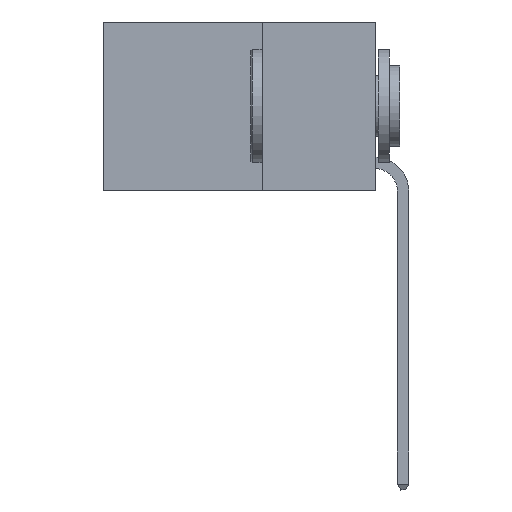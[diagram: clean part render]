
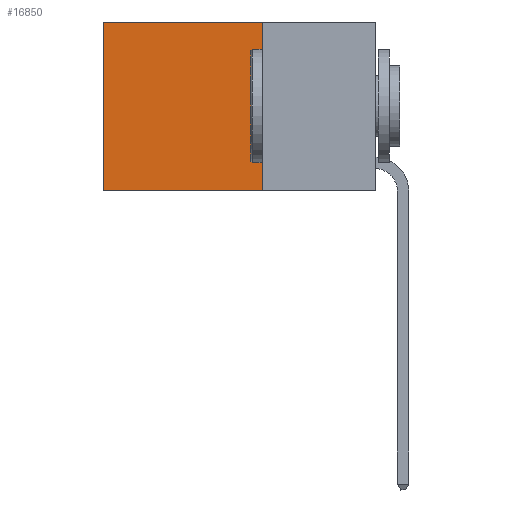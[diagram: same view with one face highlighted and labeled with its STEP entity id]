
A CAD part, left-side view. The second image highlights one B-rep face of the part: STEP entity #16850.
In plain terms, the highlighted planar face has unit normal (-1, 0, 0).
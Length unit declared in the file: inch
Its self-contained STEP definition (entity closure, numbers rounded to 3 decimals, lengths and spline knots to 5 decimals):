
#1317 = EDGE_CURVE ( 'NONE', #27462, #2827, #13480, .T. ) ;
#1613 = EDGE_CURVE ( 'NONE', #23934, #27462, #19766, .T. ) ;
#2827 = VERTEX_POINT ( 'NONE', #24064 ) ;
#3858 = CARTESIAN_POINT ( 'NONE',  ( 0.2625, 0.25, 0. ) ) ;
#4272 = LINE ( 'NONE', #3858, #9560 ) ;
#5053 = VECTOR ( 'NONE', #24504, 39.37008 ) ;
#6585 = DIRECTION ( 'NONE',  ( 0., 0., -1. ) ) ;
#6902 = ORIENTED_EDGE ( 'NONE', *, *, #8691, .T. ) ;
#7244 = CARTESIAN_POINT ( 'NONE',  ( 0.2625, 0.6, 0. ) ) ;
#8462 = DIRECTION ( 'NONE',  ( 0., 0., -1. ) ) ;
#8691 = EDGE_CURVE ( 'NONE', #23934, #18591, #4272, .T. ) ;
#9006 = PLANE ( 'NONE',  #9726 ) ;
#9560 = VECTOR ( 'NONE', #14703, 39.37008 ) ;
#9579 = VECTOR ( 'NONE', #8462, 39.37008 ) ;
#9649 = CARTESIAN_POINT ( 'NONE',  ( 0.2625, 0.6, 0. ) ) ;
#9726 = AXIS2_PLACEMENT_3D ( 'NONE', #11151, #21744, #6585 ) ;
#11151 = CARTESIAN_POINT ( 'NONE',  ( 0.2625, 0.25, 0. ) ) ;
#13480 = LINE ( 'NONE', #16049, #5053 ) ;
#13597 = CARTESIAN_POINT ( 'NONE',  ( 0.2625, 0.25, 0. ) ) ;
#14356 = DIRECTION ( 'NONE',  ( 0., 0., -1. ) ) ;
#14703 = DIRECTION ( 'NONE',  ( 0., 1., 0. ) ) ;
#14743 = ORIENTED_EDGE ( 'NONE', *, *, #21431, .T. ) ;
#15026 = CARTESIAN_POINT ( 'NONE',  ( 0.2625, 0.25, 0. ) ) ;
#16049 = CARTESIAN_POINT ( 'NONE',  ( 0.2625, 0.25, -0.37 ) ) ;
#16228 = LINE ( 'NONE', #9649, #24456 ) ;
#16850 = ADVANCED_FACE ( 'NONE', ( #24316 ), #9006, .F. ) ;
#16988 = EDGE_LOOP ( 'NONE', ( #14743, #19838, #17012, #6902 ) ) ;
#17012 = ORIENTED_EDGE ( 'NONE', *, *, #1613, .F. ) ;
#18591 = VERTEX_POINT ( 'NONE', #7244 ) ;
#19766 = LINE ( 'NONE', #15026, #9579 ) ;
#19838 = ORIENTED_EDGE ( 'NONE', *, *, #1317, .F. ) ;
#19950 = CARTESIAN_POINT ( 'NONE',  ( 0.2625, 0.25, -0.37 ) ) ;
#21431 = EDGE_CURVE ( 'NONE', #18591, #2827, #16228, .T. ) ;
#21744 = DIRECTION ( 'NONE',  ( 1., 0., 0. ) ) ;
#23934 = VERTEX_POINT ( 'NONE', #13597 ) ;
#24064 = CARTESIAN_POINT ( 'NONE',  ( 0.2625, 0.6, -0.37 ) ) ;
#24316 = FACE_OUTER_BOUND ( 'NONE', #16988, .T. ) ;
#24456 = VECTOR ( 'NONE', #14356, 39.37008 ) ;
#24504 = DIRECTION ( 'NONE',  ( 0., 1., 0. ) ) ;
#27462 = VERTEX_POINT ( 'NONE', #19950 ) ;
